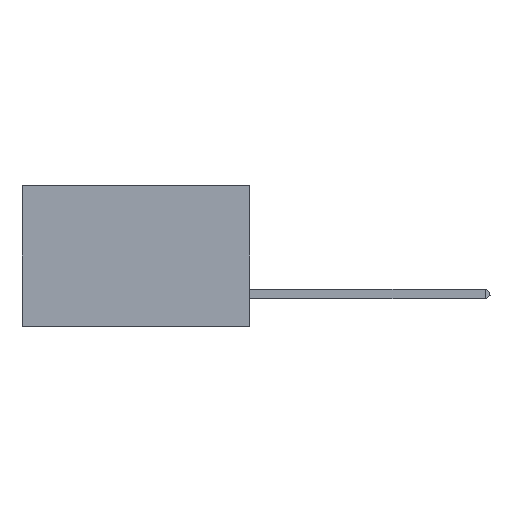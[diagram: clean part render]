
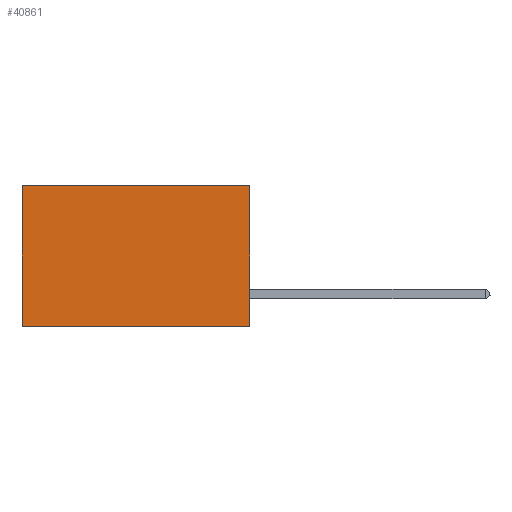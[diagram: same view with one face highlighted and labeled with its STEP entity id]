
A CAD part, left-side view. The second image highlights one B-rep face of the part: STEP entity #40861.
In plain terms, the highlighted planar face has unit normal (-1, 0, 0).
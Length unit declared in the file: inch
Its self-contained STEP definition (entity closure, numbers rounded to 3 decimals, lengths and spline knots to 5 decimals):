
#1000 = EDGE_LOOP ( 'NONE', ( #19985, #21258, #40119, #28886 ) ) ;
#1374 = CARTESIAN_POINT ( 'NONE',  ( 0.2875, 0., 0. ) ) ;
#3296 = CARTESIAN_POINT ( 'NONE',  ( 0.2875, 0.6, 0. ) ) ;
#5021 = DIRECTION ( 'NONE',  ( 0., 1., 0. ) ) ;
#6848 = PLANE ( 'NONE',  #39926 ) ;
#6869 = LINE ( 'NONE', #1374, #18572 ) ;
#8960 = VERTEX_POINT ( 'NONE', #45672 ) ;
#13216 = CARTESIAN_POINT ( 'NONE',  ( 0.2875, 0., -0.37 ) ) ;
#17720 = DIRECTION ( 'NONE',  ( 0., 0., -1. ) ) ;
#18572 = VECTOR ( 'NONE', #19573, 39.37008 ) ;
#18864 = EDGE_CURVE ( 'NONE', #38218, #8960, #44937, .T. ) ;
#18963 = VECTOR ( 'NONE', #17720, 39.37008 ) ;
#19328 = VECTOR ( 'NONE', #5021, 39.37008 ) ;
#19573 = DIRECTION ( 'NONE',  ( 0., 1., 0. ) ) ;
#19985 = ORIENTED_EDGE ( 'NONE', *, *, #18864, .T. ) ;
#21115 = CARTESIAN_POINT ( 'NONE',  ( 0.2875, 0., 0. ) ) ;
#21258 = ORIENTED_EDGE ( 'NONE', *, *, #39616, .F. ) ;
#22689 = VERTEX_POINT ( 'NONE', #21115 ) ;
#24849 = LINE ( 'NONE', #29192, #18963 ) ;
#25878 = VERTEX_POINT ( 'NONE', #28853 ) ;
#28853 = CARTESIAN_POINT ( 'NONE',  ( 0.2875, 0., -0.37 ) ) ;
#28886 = ORIENTED_EDGE ( 'NONE', *, *, #36130, .T. ) ;
#29192 = CARTESIAN_POINT ( 'NONE',  ( 0.2875, 0., 0. ) ) ;
#29468 = DIRECTION ( 'NONE',  ( 1., 0., 0. ) ) ;
#33618 = FACE_OUTER_BOUND ( 'NONE', #1000, .T. ) ;
#36130 = EDGE_CURVE ( 'NONE', #22689, #38218, #6869, .T. ) ;
#36909 = DIRECTION ( 'NONE',  ( 0., 0., -1. ) ) ;
#38218 = VERTEX_POINT ( 'NONE', #3296 ) ;
#39616 = EDGE_CURVE ( 'NONE', #25878, #8960, #39934, .T. ) ;
#39926 = AXIS2_PLACEMENT_3D ( 'NONE', #40616, #29468, #44425 ) ;
#39934 = LINE ( 'NONE', #13216, #19328 ) ;
#40119 = ORIENTED_EDGE ( 'NONE', *, *, #40506, .F. ) ;
#40506 = EDGE_CURVE ( 'NONE', #22689, #25878, #24849, .T. ) ;
#40616 = CARTESIAN_POINT ( 'NONE',  ( 0.2875, 0., 0. ) ) ;
#40861 = ADVANCED_FACE ( 'NONE', ( #33618 ), #6848, .F. ) ;
#44425 = DIRECTION ( 'NONE',  ( 0., 0., -1. ) ) ;
#44937 = LINE ( 'NONE', #44970, #46664 ) ;
#44970 = CARTESIAN_POINT ( 'NONE',  ( 0.2875, 0.6, 0. ) ) ;
#45672 = CARTESIAN_POINT ( 'NONE',  ( 0.2875, 0.6, -0.37 ) ) ;
#46664 = VECTOR ( 'NONE', #36909, 39.37008 ) ;
